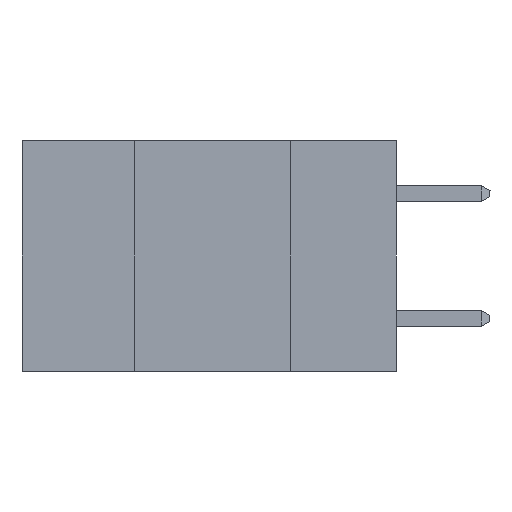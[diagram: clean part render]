
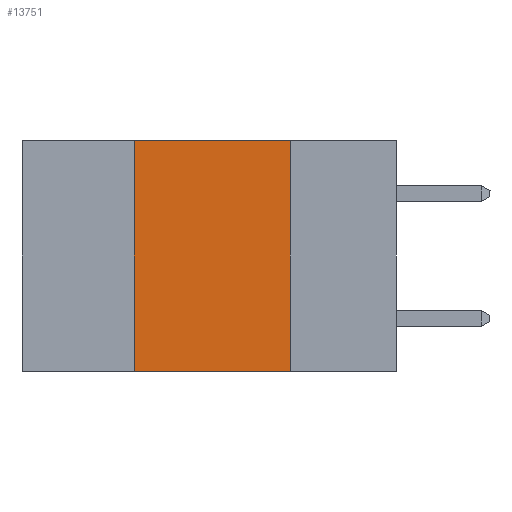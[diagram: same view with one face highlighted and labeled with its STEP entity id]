
A CAD part, left-side view. The second image highlights one B-rep face of the part: STEP entity #13751.
In plain terms, the highlighted planar face has unit normal (-1, 0, 0).
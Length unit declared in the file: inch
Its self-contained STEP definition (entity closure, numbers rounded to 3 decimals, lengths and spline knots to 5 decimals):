
#2400 = CARTESIAN_POINT ( 'NONE',  ( 0., 0.6, 0. ) ) ;
#3161 = EDGE_CURVE ( 'NONE', #18361, #17583, #17440, .T. ) ;
#3409 = CARTESIAN_POINT ( 'NONE',  ( 0., 0.6, 0. ) ) ;
#3718 = CARTESIAN_POINT ( 'NONE',  ( 0., 0.17, -0.37 ) ) ;
#4560 = LINE ( 'NONE', #3409, #11802 ) ;
#5995 = PLANE ( 'NONE',  #22469 ) ;
#6029 = VECTOR ( 'NONE', #8600, 39.37008 ) ;
#6530 = ORIENTED_EDGE ( 'NONE', *, *, #11093, .F. ) ;
#6757 = EDGE_CURVE ( 'NONE', #16900, #11770, #4560, .T. ) ;
#6900 = CARTESIAN_POINT ( 'NONE',  ( 0., 0.6, -0.37 ) ) ;
#6988 = DIRECTION ( 'NONE',  ( 0., -1., 0. ) ) ;
#7175 = LINE ( 'NONE', #22127, #16075 ) ;
#8600 = DIRECTION ( 'NONE',  ( 0., 0., -1. ) ) ;
#10833 = DIRECTION ( 'NONE',  ( 0., -1., 0. ) ) ;
#10845 = CARTESIAN_POINT ( 'NONE',  ( 0., 0.42, 0. ) ) ;
#11093 = EDGE_CURVE ( 'NONE', #11770, #17583, #21295, .T. ) ;
#11373 = DIRECTION ( 'NONE',  ( 0., 0., -1. ) ) ;
#11770 = VERTEX_POINT ( 'NONE', #22611 ) ;
#11802 = VECTOR ( 'NONE', #6988, 39.37008 ) ;
#12322 = CARTESIAN_POINT ( 'NONE',  ( 0., 0.42, -0.37 ) ) ;
#12708 = VECTOR ( 'NONE', #10833, 39.37008 ) ;
#13751 = ADVANCED_FACE ( 'NONE', ( #13948 ), #5995, .F. ) ;
#13948 = FACE_OUTER_BOUND ( 'NONE', #16642, .T. ) ;
#15025 = DIRECTION ( 'NONE',  ( 0., 0., 1. ) ) ;
#15955 = ORIENTED_EDGE ( 'NONE', *, *, #6757, .F. ) ;
#16075 = VECTOR ( 'NONE', #15025, 39.37008 ) ;
#16483 = EDGE_CURVE ( 'NONE', #18361, #16900, #7175, .T. ) ;
#16642 = EDGE_LOOP ( 'NONE', ( #6530, #15955, #20335, #21520 ) ) ;
#16900 = VERTEX_POINT ( 'NONE', #10845 ) ;
#17440 = LINE ( 'NONE', #6900, #12708 ) ;
#17442 = CARTESIAN_POINT ( 'NONE',  ( 0., 0.17, 0. ) ) ;
#17583 = VERTEX_POINT ( 'NONE', #3718 ) ;
#18361 = VERTEX_POINT ( 'NONE', #12322 ) ;
#20335 = ORIENTED_EDGE ( 'NONE', *, *, #16483, .F. ) ;
#21295 = LINE ( 'NONE', #17442, #6029 ) ;
#21520 = ORIENTED_EDGE ( 'NONE', *, *, #3161, .T. ) ;
#21958 = DIRECTION ( 'NONE',  ( 1., 0., 0. ) ) ;
#22127 = CARTESIAN_POINT ( 'NONE',  ( 0., 0.42, 0. ) ) ;
#22469 = AXIS2_PLACEMENT_3D ( 'NONE', #2400, #21958, #11373 ) ;
#22611 = CARTESIAN_POINT ( 'NONE',  ( 0., 0.17, 0. ) ) ;
